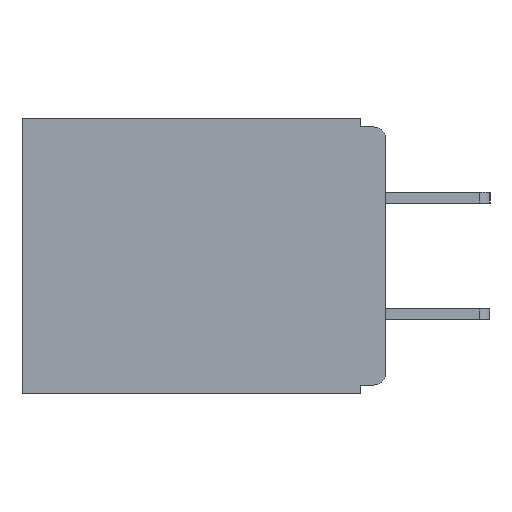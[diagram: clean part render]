
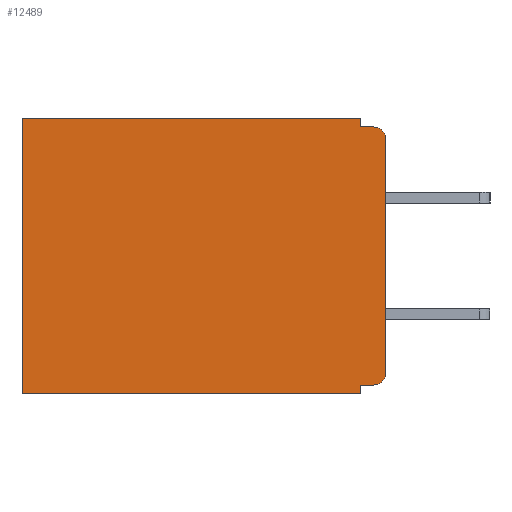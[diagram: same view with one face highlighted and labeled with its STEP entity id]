
A CAD part, left-side view. The second image highlights one B-rep face of the part: STEP entity #12489.
In plain terms, the highlighted planar face has unit normal (-1, 0, 0).
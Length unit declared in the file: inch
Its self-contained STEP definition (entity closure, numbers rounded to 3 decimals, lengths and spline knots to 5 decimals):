
#694 = CARTESIAN_POINT ( 'NONE',  ( 0.3, 0.031, 0. ) ) ;
#1127 = EDGE_CURVE ( 'NONE', #7896, #21890, #22735, .T. ) ;
#1198 = DIRECTION ( 'NONE',  ( 0., 0., -1. ) ) ;
#1375 = LINE ( 'NONE', #3083, #10517 ) ;
#1573 = DIRECTION ( 'NONE',  ( 0., -1., 0. ) ) ;
#1647 = CARTESIAN_POINT ( 'NONE',  ( 0.3, 0., -0.01 ) ) ;
#1781 = CARTESIAN_POINT ( 'NONE',  ( 0.3, 0., -0.305 ) ) ;
#2115 = VECTOR ( 'NONE', #11553, 39.37008 ) ;
#2148 = CARTESIAN_POINT ( 'NONE',  ( 0.3, 0.031, 0. ) ) ;
#2160 = VECTOR ( 'NONE', #10605, 39.37008 ) ;
#2219 = CARTESIAN_POINT ( 'NONE',  ( 0.3, 0., -0.33 ) ) ;
#2734 = LINE ( 'NONE', #10582, #2160 ) ;
#2916 = CARTESIAN_POINT ( 'NONE',  ( 0.3, 0.015, -0.32 ) ) ;
#3045 = CARTESIAN_POINT ( 'NONE',  ( 0.3, 0., -0.33 ) ) ;
#3083 = CARTESIAN_POINT ( 'NONE',  ( 0.3, 0.437, -0.33 ) ) ;
#3088 = DIRECTION ( 'NONE',  ( 0., 1., 0. ) ) ;
#3237 = VERTEX_POINT ( 'NONE', #694 ) ;
#3689 = AXIS2_PLACEMENT_3D ( 'NONE', #2219, #22304, #11378 ) ;
#3799 = ORIENTED_EDGE ( 'NONE', *, *, #6619, .F. ) ;
#3877 = FACE_OUTER_BOUND ( 'NONE', #10607, .T. ) ;
#3972 = CARTESIAN_POINT ( 'NONE',  ( 0.3, 0.031, -0.32 ) ) ;
#4622 = AXIS2_PLACEMENT_3D ( 'NONE', #23027, #12151, #1198 ) ;
#4902 = DIRECTION ( 'NONE',  ( 0., 0., -1. ) ) ;
#5858 = LINE ( 'NONE', #20688, #14971 ) ;
#6619 = EDGE_CURVE ( 'NONE', #6972, #21203, #2734, .T. ) ;
#6972 = VERTEX_POINT ( 'NONE', #3972 ) ;
#7160 = ORIENTED_EDGE ( 'NONE', *, *, #7269, .F. ) ;
#7269 = EDGE_CURVE ( 'NONE', #20080, #21953, #21016, .T. ) ;
#7863 = EDGE_CURVE ( 'NONE', #3237, #7896, #21810, .T. ) ;
#7896 = VERTEX_POINT ( 'NONE', #22230 ) ;
#8552 = ORIENTED_EDGE ( 'NONE', *, *, #16269, .T. ) ;
#8642 = VERTEX_POINT ( 'NONE', #2916 ) ;
#8819 = CARTESIAN_POINT ( 'NONE',  ( 0.3, 0., -0.025 ) ) ;
#9863 = VECTOR ( 'NONE', #12175, 39.37008 ) ;
#10301 = DIRECTION ( 'NONE',  ( -1., 0., 0. ) ) ;
#10342 = CARTESIAN_POINT ( 'NONE',  ( 0.3, 0., -0.32 ) ) ;
#10517 = VECTOR ( 'NONE', #4902, 39.37008 ) ;
#10582 = CARTESIAN_POINT ( 'NONE',  ( 0.3, 0.031, -0.33 ) ) ;
#10605 = DIRECTION ( 'NONE',  ( 0., 0., -1. ) ) ;
#10607 = EDGE_LOOP ( 'NONE', ( #7160, #8552, #11055, #14733, #22321, #11150, #17916, #3799, #15478, #21845 ) ) ;
#11055 = ORIENTED_EDGE ( 'NONE', *, *, #1127, .F. ) ;
#11150 = ORIENTED_EDGE ( 'NONE', *, *, #17032, .T. ) ;
#11378 = DIRECTION ( 'NONE',  ( 0., 0., -1. ) ) ;
#11553 = DIRECTION ( 'NONE',  ( 0., 0., -1. ) ) ;
#12026 = AXIS2_PLACEMENT_3D ( 'NONE', #21262, #10301, #23007 ) ;
#12151 = DIRECTION ( 'NONE',  ( -1., 0., 0. ) ) ;
#12175 = DIRECTION ( 'NONE',  ( 0., 1., 0. ) ) ;
#12489 = ADVANCED_FACE ( 'NONE', ( #3877 ), #13136, .F. ) ;
#12653 = VECTOR ( 'NONE', #14881, 39.37008 ) ;
#13108 = CIRCLE ( 'NONE', #12026, 0.015 ) ;
#13136 = PLANE ( 'NONE',  #3689 ) ;
#13818 = EDGE_CURVE ( 'NONE', #8642, #21953, #14085, .T. ) ;
#14008 = CARTESIAN_POINT ( 'NONE',  ( 0.3, 0., -0.33 ) ) ;
#14085 = CIRCLE ( 'NONE', #4622, 0.015 ) ;
#14733 = ORIENTED_EDGE ( 'NONE', *, *, #7863, .F. ) ;
#14881 = DIRECTION ( 'NONE',  ( 0., 0., -1. ) ) ;
#14971 = VECTOR ( 'NONE', #22434, 39.37008 ) ;
#15478 = ORIENTED_EDGE ( 'NONE', *, *, #19989, .F. ) ;
#15809 = LINE ( 'NONE', #10342, #9863 ) ;
#16215 = CARTESIAN_POINT ( 'NONE',  ( 0.3, 0.015, -0.01 ) ) ;
#16219 = VERTEX_POINT ( 'NONE', #22783 ) ;
#16269 = EDGE_CURVE ( 'NONE', #20080, #21890, #13108, .T. ) ;
#16544 = CARTESIAN_POINT ( 'NONE',  ( 0.3, 0.437, 0. ) ) ;
#17032 = EDGE_CURVE ( 'NONE', #23401, #16219, #1375, .T. ) ;
#17324 = VECTOR ( 'NONE', #1573, 39.37008 ) ;
#17916 = ORIENTED_EDGE ( 'NONE', *, *, #18873, .F. ) ;
#18873 = EDGE_CURVE ( 'NONE', #21203, #16219, #19328, .T. ) ;
#19306 = EDGE_CURVE ( 'NONE', #3237, #23401, #5858, .T. ) ;
#19328 = LINE ( 'NONE', #14008, #19918 ) ;
#19918 = VECTOR ( 'NONE', #3088, 39.37008 ) ;
#19989 = EDGE_CURVE ( 'NONE', #8642, #6972, #15809, .T. ) ;
#20080 = VERTEX_POINT ( 'NONE', #8819 ) ;
#20688 = CARTESIAN_POINT ( 'NONE',  ( 0.3, 0., 0. ) ) ;
#21016 = LINE ( 'NONE', #3045, #2115 ) ;
#21203 = VERTEX_POINT ( 'NONE', #22847 ) ;
#21262 = CARTESIAN_POINT ( 'NONE',  ( 0.3, 0.015, -0.025 ) ) ;
#21810 = LINE ( 'NONE', #2148, #12653 ) ;
#21845 = ORIENTED_EDGE ( 'NONE', *, *, #13818, .T. ) ;
#21890 = VERTEX_POINT ( 'NONE', #16215 ) ;
#21953 = VERTEX_POINT ( 'NONE', #1781 ) ;
#22230 = CARTESIAN_POINT ( 'NONE',  ( 0.3, 0.031, -0.01 ) ) ;
#22304 = DIRECTION ( 'NONE',  ( 1., 0., 0. ) ) ;
#22321 = ORIENTED_EDGE ( 'NONE', *, *, #19306, .T. ) ;
#22434 = DIRECTION ( 'NONE',  ( 0., 1., 0. ) ) ;
#22735 = LINE ( 'NONE', #1647, #17324 ) ;
#22783 = CARTESIAN_POINT ( 'NONE',  ( 0.3, 0.437, -0.33 ) ) ;
#22847 = CARTESIAN_POINT ( 'NONE',  ( 0.3, 0.031, -0.33 ) ) ;
#23007 = DIRECTION ( 'NONE',  ( 0., 0., -1. ) ) ;
#23027 = CARTESIAN_POINT ( 'NONE',  ( 0.3, 0.015, -0.305 ) ) ;
#23401 = VERTEX_POINT ( 'NONE', #16544 ) ;
